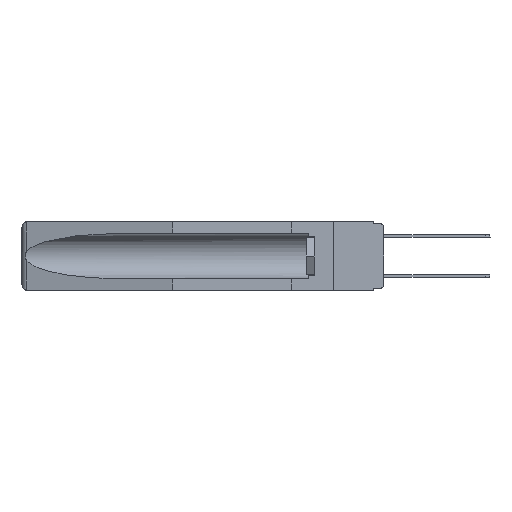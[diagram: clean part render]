
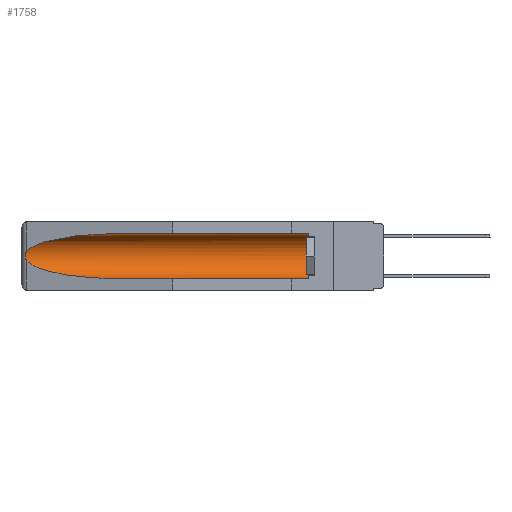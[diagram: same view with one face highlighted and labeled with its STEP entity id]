
A CAD part, left-side view. The second image highlights one B-rep face of the part: STEP entity #1758.
In plain terms, the highlighted cylindrical face has radius 2.857 mm (diameter 5.715 mm), a partial arc.
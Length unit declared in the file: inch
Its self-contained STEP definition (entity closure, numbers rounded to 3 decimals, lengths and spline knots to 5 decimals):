
#535 = CARTESIAN_POINT ( 'NONE',  ( 0.2675, 1.53308, -0.17534 ) ) ;
#1001 = VERTEX_POINT ( 'NONE', #6663 ) ;
#1758 = ADVANCED_FACE ( 'NONE', ( #12780 ), #12279, .F. ) ;
#2161 = CARTESIAN_POINT ( 'NONE',  ( 0.26537, 1.52718, -0.14972 ) ) ;
#2232 = CARTESIAN_POINT ( 'NONE',  ( 0.2673, 1.53269, -0.17917 ) ) ;
#2617 = LINE ( 'NONE', #6788, #10577 ) ;
#2811 = EDGE_CURVE ( 'NONE', #12266, #18566, #19250, .T. ) ;
#3179 = CARTESIAN_POINT ( 'NONE',  ( 0.25451, 1.48313, -0.24835 ) ) ;
#3314 = CARTESIAN_POINT ( 'NONE',  ( 0.26537, 1.52718, -0.19328 ) ) ;
#3333 = DIRECTION ( 'NONE',  ( 0., 1., 0. ) ) ;
#3478 = CARTESIAN_POINT ( 'NONE',  ( 0.155, 0.126, -0.284 ) ) ;
#3591 = CARTESIAN_POINT ( 'NONE',  ( 0.26654, 1.53092, -0.15636 ) ) ;
#3655 = CARTESIAN_POINT ( 'NONE',  ( 0.26537, 1.52718, -0.19328 ) ) ;
#3862 = ORIENTED_EDGE ( 'NONE', *, *, #12800, .T. ) ;
#4270 = CARTESIAN_POINT ( 'NONE',  ( 0.155, -0.30754, -0.059 ) ) ;
#5552 = DIRECTION ( 'NONE',  ( 0., 0., 1. ) ) ;
#5925 = ORIENTED_EDGE ( 'NONE', *, *, #15551, .T. ) ;
#6496 = CARTESIAN_POINT ( 'NONE',  ( 0.155, 1.07973, -0.059 ) ) ;
#6663 = CARTESIAN_POINT ( 'NONE',  ( 0.26537, 1.52718, -0.14972 ) ) ;
#6701 = CARTESIAN_POINT ( 'NONE',  ( 0.26537, 1.52718, -0.14972 ) ) ;
#6788 = CARTESIAN_POINT ( 'NONE',  ( 0.155, -0.30754, -0.284 ) ) ;
#7372 = ORIENTED_EDGE ( 'NONE', *, *, #12705, .T. ) ;
#7395 = CARTESIAN_POINT ( 'NONE',  ( 0.155, 1.07973, -0.284 ) ) ;
#7496 = DIRECTION ( 'NONE',  ( 0., 0., 1. ) ) ;
#8106 =( BOUNDED_CURVE ( )  B_SPLINE_CURVE ( 3, ( #3314, #3179, #9933, #19688 ),
 .UNSPECIFIED., .F., .F. ) 
 B_SPLINE_CURVE_WITH_KNOTS ( ( 4, 4 ),
 ( 0.1948, 1.5708 ),
 .UNSPECIFIED. ) 
 CURVE ( )  GEOMETRIC_REPRESENTATION_ITEM ( )  RATIONAL_B_SPLINE_CURVE ( ( 1., 0.848, 0.848, 1. ) ) 
 REPRESENTATION_ITEM ( '' )  );
#8482 = CARTESIAN_POINT ( 'NONE',  ( 0.26597, 1.5296, -0.19026 ) ) ;
#8495 = CARTESIAN_POINT ( 'NONE',  ( 0.155, 1.07973, -0.059 ) ) ;
#8783 = DIRECTION ( 'NONE',  ( 0., -1., 0. ) ) ;
#9114 = VERTEX_POINT ( 'NONE', #7395 ) ;
#9256 = DIRECTION ( 'NONE',  ( 0., 1., 0. ) ) ;
#9488 = AXIS2_PLACEMENT_3D ( 'NONE', #13874, #12248, #7496 ) ;
#9933 = CARTESIAN_POINT ( 'NONE',  ( 0.21114, 1.30732, -0.284 ) ) ;
#10577 = VECTOR ( 'NONE', #3333, 39.37008 ) ;
#10614 = B_SPLINE_CURVE_WITH_KNOTS ( 'NONE', 3,
 ( #2161, #13645, #3591, #18622, #13497, #535, #2232, #16689, #8482, #3655 ),
 .UNSPECIFIED., .F., .F.,
 ( 4, 2, 2, 2, 4 ),
 ( 0., 0.00029, 0.00058, 0.00087, 0.00117 ),
 .UNSPECIFIED. ) ;
#11096 = AXIS2_PLACEMENT_3D ( 'NONE', #15413, #8783, #5552 ) ;
#11833 = ORIENTED_EDGE ( 'NONE', *, *, #17030, .T. ) ;
#12157 = VECTOR ( 'NONE', #9256, 39.37008 ) ;
#12248 = DIRECTION ( 'NONE',  ( 0., 1., 0. ) ) ;
#12266 = VERTEX_POINT ( 'NONE', #20266 ) ;
#12279 = CYLINDRICAL_SURFACE ( 'NONE', #9488, 0.1125 ) ;
#12705 = EDGE_CURVE ( 'NONE', #18566, #1001, #12850, .T. ) ;
#12780 = FACE_OUTER_BOUND ( 'NONE', #13578, .T. ) ;
#12800 = EDGE_CURVE ( 'NONE', #19910, #12266, #17304, .T. ) ;
#12850 =( BOUNDED_CURVE ( )  B_SPLINE_CURVE ( 3, ( #8495, #13440, #18405, #6701 ),
 .UNSPECIFIED., .F., .F. ) 
 B_SPLINE_CURVE_WITH_KNOTS ( ( 4, 4 ),
 ( 4.71239, 6.08839 ),
 .UNSPECIFIED. ) 
 CURVE ( )  GEOMETRIC_REPRESENTATION_ITEM ( )  RATIONAL_B_SPLINE_CURVE ( ( 1., 0.848, 0.848, 1. ) ) 
 REPRESENTATION_ITEM ( '' )  );
#13440 = CARTESIAN_POINT ( 'NONE',  ( 0.21114, 1.30732, -0.059 ) ) ;
#13497 = CARTESIAN_POINT ( 'NONE',  ( 0.2675, 1.53308, -0.16763 ) ) ;
#13578 = EDGE_LOOP ( 'NONE', ( #7372, #11833, #5925, #19516, #3862, #20023 ) ) ;
#13645 = CARTESIAN_POINT ( 'NONE',  ( 0.26597, 1.52961, -0.15275 ) ) ;
#13874 = CARTESIAN_POINT ( 'NONE',  ( 0.155, -0.30754, -0.1715 ) ) ;
#15413 = CARTESIAN_POINT ( 'NONE',  ( 0.155, 0.126, -0.1715 ) ) ;
#15428 = VERTEX_POINT ( 'NONE', #20837 ) ;
#15551 = EDGE_CURVE ( 'NONE', #15428, #9114, #8106, .T. ) ;
#16689 = CARTESIAN_POINT ( 'NONE',  ( 0.26655, 1.53094, -0.18657 ) ) ;
#17030 = EDGE_CURVE ( 'NONE', #1001, #15428, #10614, .T. ) ;
#17304 = CIRCLE ( 'NONE', #11096, 0.1125 ) ;
#18129 = EDGE_CURVE ( 'NONE', #19910, #9114, #2617, .T. ) ;
#18405 = CARTESIAN_POINT ( 'NONE',  ( 0.25451, 1.48313, -0.09465 ) ) ;
#18566 = VERTEX_POINT ( 'NONE', #6496 ) ;
#18622 = CARTESIAN_POINT ( 'NONE',  ( 0.2673, 1.5327, -0.16383 ) ) ;
#19250 = LINE ( 'NONE', #4270, #12157 ) ;
#19516 = ORIENTED_EDGE ( 'NONE', *, *, #18129, .F. ) ;
#19688 = CARTESIAN_POINT ( 'NONE',  ( 0.155, 1.07973, -0.284 ) ) ;
#19910 = VERTEX_POINT ( 'NONE', #3478 ) ;
#20023 = ORIENTED_EDGE ( 'NONE', *, *, #2811, .T. ) ;
#20266 = CARTESIAN_POINT ( 'NONE',  ( 0.155, 0.126, -0.059 ) ) ;
#20837 = CARTESIAN_POINT ( 'NONE',  ( 0.26537, 1.52718, -0.19328 ) ) ;
